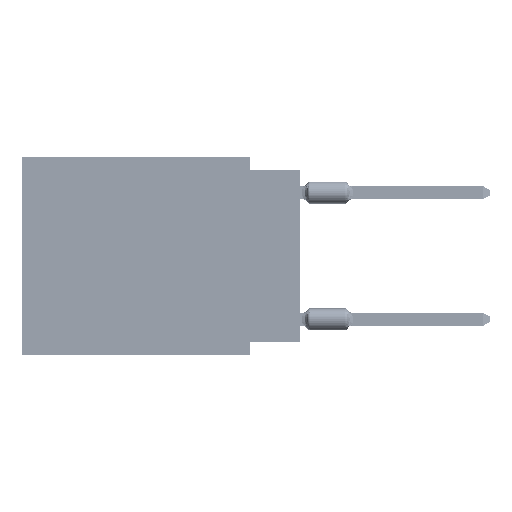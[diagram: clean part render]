
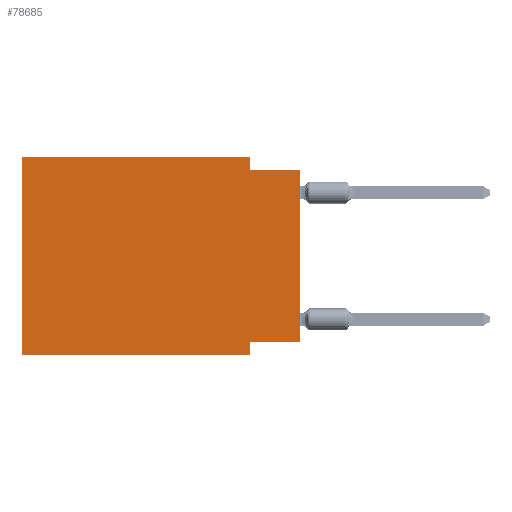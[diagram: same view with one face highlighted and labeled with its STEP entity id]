
A CAD part, left-side view. The second image highlights one B-rep face of the part: STEP entity #78685.
In plain terms, the highlighted planar face has unit normal (-1, 0, 0).
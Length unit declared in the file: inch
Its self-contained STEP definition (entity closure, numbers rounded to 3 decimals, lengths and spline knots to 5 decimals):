
#1282 = DIRECTION ( 'NONE',  ( 0., 0., 1. ) ) ;
#2541 = CARTESIAN_POINT ( 'NONE',  ( 0., 0., -0.025 ) ) ;
#5071 = LINE ( 'NONE', #51751, #72430 ) ;
#6737 = ORIENTED_EDGE ( 'NONE', *, *, #27333, .F. ) ;
#8463 = CARTESIAN_POINT ( 'NONE',  ( 0., 0.1, -0.39 ) ) ;
#12069 = VECTOR ( 'NONE', #24019, 39.37008 ) ;
#12141 = CARTESIAN_POINT ( 'NONE',  ( 0., 0.55, -0.39 ) ) ;
#12591 = DIRECTION ( 'NONE',  ( 0., -1., 0. ) ) ;
#13156 = AXIS2_PLACEMENT_3D ( 'NONE', #31510, #37384, #31955 ) ;
#15712 = CARTESIAN_POINT ( 'NONE',  ( 0., 0.55, 0. ) ) ;
#16378 = CARTESIAN_POINT ( 'NONE',  ( 0., 0.55, 0. ) ) ;
#16880 = CARTESIAN_POINT ( 'NONE',  ( 0., 0.1, -0.025 ) ) ;
#18105 = DIRECTION ( 'NONE',  ( 0., -1., 0. ) ) ;
#22567 = ORIENTED_EDGE ( 'NONE', *, *, #34152, .F. ) ;
#24019 = DIRECTION ( 'NONE',  ( 0., 0., 1. ) ) ;
#24263 = VERTEX_POINT ( 'NONE', #33617 ) ;
#24635 = ORIENTED_EDGE ( 'NONE', *, *, #60390, .F. ) ;
#25358 = CARTESIAN_POINT ( 'NONE',  ( 0., 0.1, -0.365 ) ) ;
#27333 = EDGE_CURVE ( 'NONE', #82532, #63139, #69937, .T. ) ;
#31510 = CARTESIAN_POINT ( 'NONE',  ( 0., 0.55, 0. ) ) ;
#31955 = DIRECTION ( 'NONE',  ( 0., 0., -1. ) ) ;
#32414 = FACE_OUTER_BOUND ( 'NONE', #72911, .T. ) ;
#33617 = CARTESIAN_POINT ( 'NONE',  ( 0., 0.55, -0.39 ) ) ;
#34152 = EDGE_CURVE ( 'NONE', #24263, #54477, #77883, .T. ) ;
#34661 = EDGE_CURVE ( 'NONE', #74372, #63626, #59356, .T. ) ;
#35493 = LINE ( 'NONE', #62839, #86327 ) ;
#35849 = DIRECTION ( 'NONE',  ( 0., 0., -1. ) ) ;
#37384 = DIRECTION ( 'NONE',  ( 1., 0., 0. ) ) ;
#38080 = CARTESIAN_POINT ( 'NONE',  ( 0., 0., -0.365 ) ) ;
#39338 = VECTOR ( 'NONE', #82924, 39.37008 ) ;
#40734 = ORIENTED_EDGE ( 'NONE', *, *, #83292, .F. ) ;
#42122 = LINE ( 'NONE', #55151, #66589 ) ;
#42664 = EDGE_CURVE ( 'NONE', #51610, #82532, #35493, .T. ) ;
#43714 = VECTOR ( 'NONE', #46324, 39.37008 ) ;
#44662 = CARTESIAN_POINT ( 'NONE',  ( 0., 0.55, 0. ) ) ;
#44965 = PLANE ( 'NONE',  #13156 ) ;
#45555 = CARTESIAN_POINT ( 'NONE',  ( 0., 0.1, 0. ) ) ;
#46324 = DIRECTION ( 'NONE',  ( 0., 0., -1. ) ) ;
#51610 = VERTEX_POINT ( 'NONE', #38080 ) ;
#51751 = CARTESIAN_POINT ( 'NONE',  ( 0., 0., -0.025 ) ) ;
#54477 = VERTEX_POINT ( 'NONE', #15712 ) ;
#55151 = CARTESIAN_POINT ( 'NONE',  ( 0., 0., 0. ) ) ;
#55589 = ORIENTED_EDGE ( 'NONE', *, *, #87705, .T. ) ;
#56815 = VECTOR ( 'NONE', #12591, 39.37008 ) ;
#58477 = CARTESIAN_POINT ( 'NONE',  ( 0., 0.1, 0. ) ) ;
#58709 = ORIENTED_EDGE ( 'NONE', *, *, #34661, .F. ) ;
#59356 = LINE ( 'NONE', #58477, #43714 ) ;
#60139 = LINE ( 'NONE', #12141, #56815 ) ;
#60390 = EDGE_CURVE ( 'NONE', #63626, #78515, #5071, .T. ) ;
#60939 = ORIENTED_EDGE ( 'NONE', *, *, #42664, .F. ) ;
#62839 = CARTESIAN_POINT ( 'NONE',  ( 0., 0., -0.365 ) ) ;
#63139 = VERTEX_POINT ( 'NONE', #66522 ) ;
#63626 = VERTEX_POINT ( 'NONE', #16880 ) ;
#65259 = LINE ( 'NONE', #16378, #39338 ) ;
#66522 = CARTESIAN_POINT ( 'NONE',  ( 0., 0.1, -0.39 ) ) ;
#66589 = VECTOR ( 'NONE', #1282, 39.37008 ) ;
#69937 = LINE ( 'NONE', #8463, #85970 ) ;
#72430 = VECTOR ( 'NONE', #18105, 39.37008 ) ;
#72723 = ORIENTED_EDGE ( 'NONE', *, *, #85445, .T. ) ;
#72911 = EDGE_LOOP ( 'NONE', ( #72723, #24635, #58709, #40734, #22567, #55589, #6737, #60939 ) ) ;
#74372 = VERTEX_POINT ( 'NONE', #45555 ) ;
#74550 = DIRECTION ( 'NONE',  ( 0., 1., 0. ) ) ;
#77883 = LINE ( 'NONE', #44662, #12069 ) ;
#78515 = VERTEX_POINT ( 'NONE', #2541 ) ;
#78685 = ADVANCED_FACE ( 'NONE', ( #32414 ), #44965, .F. ) ;
#82532 = VERTEX_POINT ( 'NONE', #25358 ) ;
#82924 = DIRECTION ( 'NONE',  ( 0., -1., 0. ) ) ;
#83292 = EDGE_CURVE ( 'NONE', #54477, #74372, #65259, .T. ) ;
#85445 = EDGE_CURVE ( 'NONE', #51610, #78515, #42122, .T. ) ;
#85970 = VECTOR ( 'NONE', #35849, 39.37008 ) ;
#86327 = VECTOR ( 'NONE', #74550, 39.37008 ) ;
#87705 = EDGE_CURVE ( 'NONE', #24263, #63139, #60139, .T. ) ;
